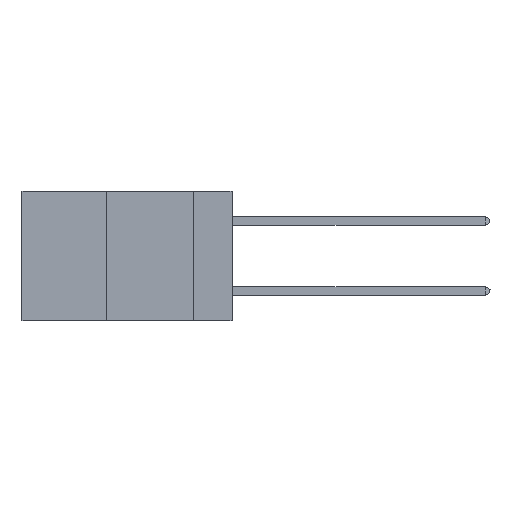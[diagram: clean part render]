
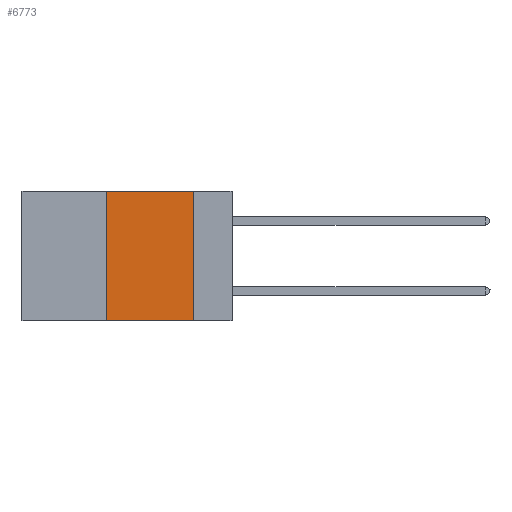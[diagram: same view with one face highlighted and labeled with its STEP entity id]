
A CAD part, left-side view. The second image highlights one B-rep face of the part: STEP entity #6773.
In plain terms, the highlighted planar face has unit normal (-1, 0, 0).
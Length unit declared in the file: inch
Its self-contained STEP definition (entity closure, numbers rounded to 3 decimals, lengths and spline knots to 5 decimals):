
#594 = DIRECTION ( 'NONE',  ( 0., -1., 0. ) ) ;
#711 = LINE ( 'NONE', #1699, #18416 ) ;
#1031 = EDGE_CURVE ( 'NONE', #7717, #8594, #12450, .T. ) ;
#1699 = CARTESIAN_POINT ( 'NONE',  ( 0., 0.11, 0. ) ) ;
#2130 = ORIENTED_EDGE ( 'NONE', *, *, #1031, .F. ) ;
#2282 = LINE ( 'NONE', #12154, #19696 ) ;
#2618 = VERTEX_POINT ( 'NONE', #15987 ) ;
#2627 = ORIENTED_EDGE ( 'NONE', *, *, #9265, .T. ) ;
#2655 = EDGE_CURVE ( 'NONE', #8968, #2618, #711, .T. ) ;
#3797 = VECTOR ( 'NONE', #6420, 39.37008 ) ;
#4873 = DIRECTION ( 'NONE',  ( 0., 0., -1. ) ) ;
#5788 = DIRECTION ( 'NONE',  ( 1., 0., 0. ) ) ;
#6078 = CARTESIAN_POINT ( 'NONE',  ( 0., 0.36, 0. ) ) ;
#6420 = DIRECTION ( 'NONE',  ( 0., -1., 0. ) ) ;
#6765 = CARTESIAN_POINT ( 'NONE',  ( 0., 0.36, 0. ) ) ;
#6773 = ADVANCED_FACE ( 'NONE', ( #15852 ), #7357, .F. ) ;
#7357 = PLANE ( 'NONE',  #14203 ) ;
#7717 = VERTEX_POINT ( 'NONE', #21820 ) ;
#8294 = LINE ( 'NONE', #16657, #3797 ) ;
#8594 = VERTEX_POINT ( 'NONE', #6765 ) ;
#8968 = VERTEX_POINT ( 'NONE', #21872 ) ;
#9145 = CARTESIAN_POINT ( 'NONE',  ( 0., 0.6, 0. ) ) ;
#9259 = VECTOR ( 'NONE', #17899, 39.37008 ) ;
#9265 = EDGE_CURVE ( 'NONE', #7717, #2618, #2282, .T. ) ;
#10690 = DIRECTION ( 'NONE',  ( 0., 0., -1. ) ) ;
#10963 = ORIENTED_EDGE ( 'NONE', *, *, #2655, .F. ) ;
#11483 = EDGE_LOOP ( 'NONE', ( #10963, #18542, #2130, #2627 ) ) ;
#12154 = CARTESIAN_POINT ( 'NONE',  ( 0., 0.6, -0.37 ) ) ;
#12450 = LINE ( 'NONE', #6078, #9259 ) ;
#14203 = AXIS2_PLACEMENT_3D ( 'NONE', #9145, #5788, #10690 ) ;
#15852 = FACE_OUTER_BOUND ( 'NONE', #11483, .T. ) ;
#15987 = CARTESIAN_POINT ( 'NONE',  ( 0., 0.11, -0.37 ) ) ;
#16657 = CARTESIAN_POINT ( 'NONE',  ( 0., 0.6, 0. ) ) ;
#17899 = DIRECTION ( 'NONE',  ( 0., 0., 1. ) ) ;
#18416 = VECTOR ( 'NONE', #4873, 39.37008 ) ;
#18542 = ORIENTED_EDGE ( 'NONE', *, *, #21595, .F. ) ;
#19696 = VECTOR ( 'NONE', #594, 39.37008 ) ;
#21595 = EDGE_CURVE ( 'NONE', #8594, #8968, #8294, .T. ) ;
#21820 = CARTESIAN_POINT ( 'NONE',  ( 0., 0.36, -0.37 ) ) ;
#21872 = CARTESIAN_POINT ( 'NONE',  ( 0., 0.11, 0. ) ) ;
